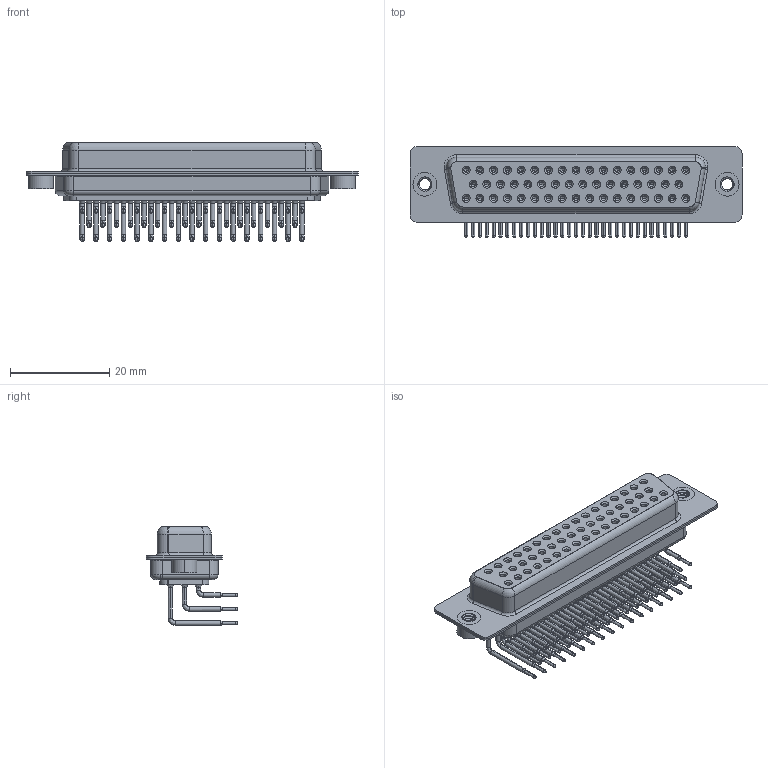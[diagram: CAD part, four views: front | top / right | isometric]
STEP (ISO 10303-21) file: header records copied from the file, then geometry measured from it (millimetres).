
FILE_DESCRIPTION (( 'STEP AP203' ), '1' );
FILE_NAME ('622-M50-660-GT2.STEP', '2018-09-25T00:05:16', ( '' ), ( '' ), 'SwSTEP 2.0', 'SolidWorks 2016', '' );
FILE_SCHEMA (( 'CONFIG_CONTROL_DESIGN' ));
Length unit declared in the file: millimetre
Products named in the file (8): 622M 4-40 Threaded Rivet; 622-M50-660-GT2; 622M Housing_50 Contacts; 622M Shell Front_50 Contacts; 622M Shell Rear_50 Contacts; 622M Contact Row 1_50 Contacts; 622M Contact Row 2_50 Contacts; 622M Contact Row 3
Assembly tree (55 placements, depth 2):
  622-M50-660-GT2
    622M Housing_50 Contacts
    622M Shell Front_50 Contacts
    622M Shell Rear_50 Contacts
    622M Contact Row 1_50 Contacts  x17
    622M Contact Row 2_50 Contacts  x16
    622M Contact Row 3  x17
    622M 4-40 Threaded Rivet  x2
Bounding box: 67 x 18.4 x 19.93 mm (x, y, z)
Volume: 6932.9 mm3; surface area: 16132.4 mm2
Topology: 55 solids, 55 shells, 2929 faces, 7437 edges, 4679 vertices
Faces by surface type: cylinder 1287, plane 817, cone 556, bspline 206, torus 63
Entity records: 33247 total; most frequent: CARTESIAN_POINT 6803, DIRECTION 5669, ORIENTED_EDGE 4628, AXIS2_PLACEMENT_3D 2399, EDGE_CURVE 2314, VERTEX_POINT 1477, CIRCLE 1340, EDGE_LOOP 1295
